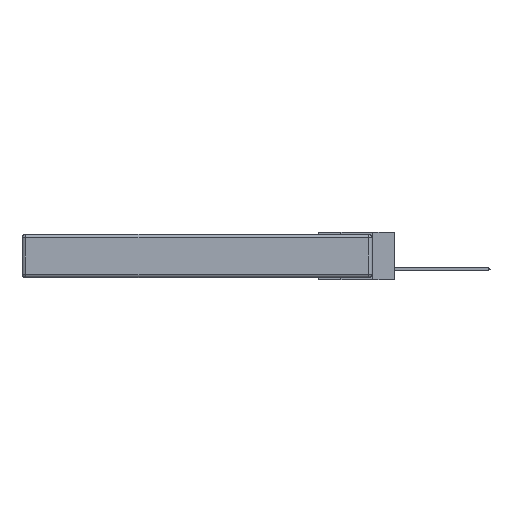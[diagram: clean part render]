
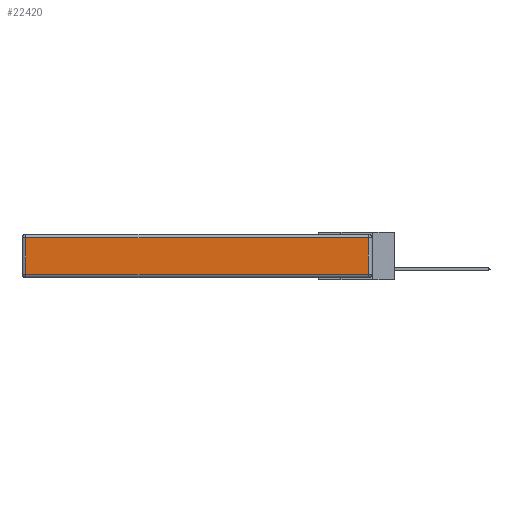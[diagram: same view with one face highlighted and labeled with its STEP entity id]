
A CAD part, left-side view. The second image highlights one B-rep face of the part: STEP entity #22420.
In plain terms, the highlighted planar face has unit normal (-1, 0, 0).
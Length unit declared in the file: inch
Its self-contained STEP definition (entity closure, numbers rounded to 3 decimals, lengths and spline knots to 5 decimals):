
#523 = DIRECTION ( 'NONE',  ( 0., 0., -1. ) ) ;
#826 = DIRECTION ( 'NONE',  ( -1., 0., 0. ) ) ;
#1604 = VECTOR ( 'NONE', #523, 39.37008 ) ;
#2009 = CARTESIAN_POINT ( 'NONE',  ( 0., 0.03, -0.313 ) ) ;
#3667 = LINE ( 'NONE', #19921, #16717 ) ;
#4784 = DIRECTION ( 'NONE',  ( 0., 0., 1. ) ) ;
#6091 = LINE ( 'NONE', #22391, #10247 ) ;
#10247 = VECTOR ( 'NONE', #24675, 39.37008 ) ;
#10309 = AXIS2_PLACEMENT_3D ( 'NONE', #13925, #826, #4784 ) ;
#12581 = CARTESIAN_POINT ( 'NONE',  ( 0., 0.03, -0.343 ) ) ;
#13152 = LINE ( 'NONE', #12581, #14843 ) ;
#13220 = ORIENTED_EDGE ( 'NONE', *, *, #23269, .T. ) ;
#13925 = CARTESIAN_POINT ( 'NONE',  ( 0., 0., -0.343 ) ) ;
#14843 = VECTOR ( 'NONE', #14944, 39.37008 ) ;
#14944 = DIRECTION ( 'NONE',  ( 0., 0., 1. ) ) ;
#16717 = VECTOR ( 'NONE', #22416, 39.37008 ) ;
#16747 = CARTESIAN_POINT ( 'NONE',  ( 0., 2.72, -0.03 ) ) ;
#17295 = VERTEX_POINT ( 'NONE', #27278 ) ;
#18094 = ORIENTED_EDGE ( 'NONE', *, *, #26035, .T. ) ;
#18319 = CARTESIAN_POINT ( 'NONE',  ( 0., 2.72, -0.343 ) ) ;
#19299 = VERTEX_POINT ( 'NONE', #2009 ) ;
#19433 = ORIENTED_EDGE ( 'NONE', *, *, #23560, .T. ) ;
#19758 = LINE ( 'NONE', #18319, #1604 ) ;
#19921 = CARTESIAN_POINT ( 'NONE',  ( 0., 0., -0.313 ) ) ;
#20495 = VERTEX_POINT ( 'NONE', #21064 ) ;
#20977 = VERTEX_POINT ( 'NONE', #16747 ) ;
#21064 = CARTESIAN_POINT ( 'NONE',  ( 0., 2.72, -0.313 ) ) ;
#22391 = CARTESIAN_POINT ( 'NONE',  ( 0., 2.75, -0.03 ) ) ;
#22416 = DIRECTION ( 'NONE',  ( 0., -1., 0. ) ) ;
#22420 = ADVANCED_FACE ( 'NONE', ( #22959 ), #26767, .T. ) ;
#22959 = FACE_OUTER_BOUND ( 'NONE', #24436, .T. ) ;
#23269 = EDGE_CURVE ( 'NONE', #17295, #20977, #6091, .T. ) ;
#23560 = EDGE_CURVE ( 'NONE', #20495, #19299, #3667, .T. ) ;
#24436 = EDGE_LOOP ( 'NONE', ( #19433, #18094, #13220, #27841 ) ) ;
#24482 = EDGE_CURVE ( 'NONE', #20977, #20495, #19758, .T. ) ;
#24675 = DIRECTION ( 'NONE',  ( 0., 1., 0. ) ) ;
#26035 = EDGE_CURVE ( 'NONE', #19299, #17295, #13152, .T. ) ;
#26767 = PLANE ( 'NONE',  #10309 ) ;
#27278 = CARTESIAN_POINT ( 'NONE',  ( 0., 0.03, -0.03 ) ) ;
#27841 = ORIENTED_EDGE ( 'NONE', *, *, #24482, .T. ) ;
